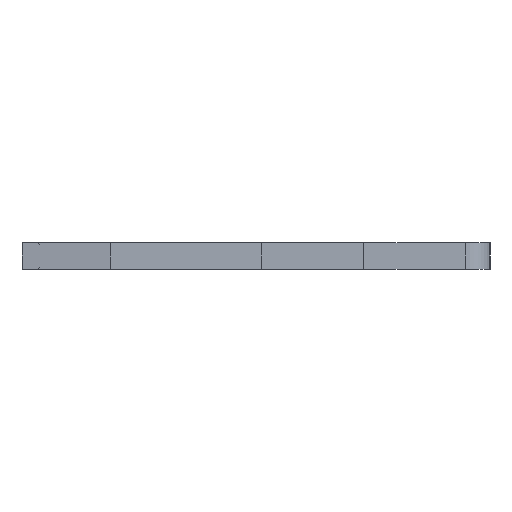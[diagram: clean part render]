
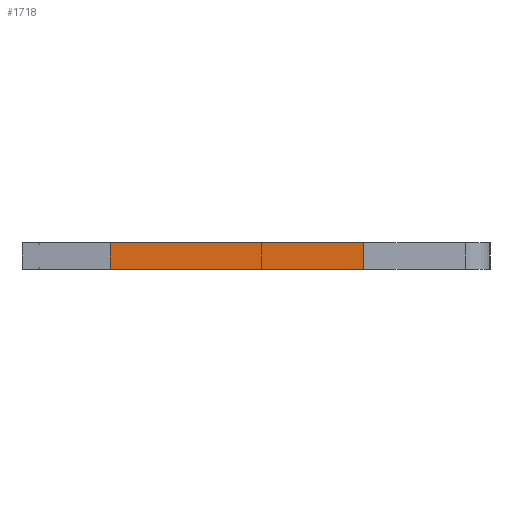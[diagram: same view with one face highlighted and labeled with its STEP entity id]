
A CAD part, left-side view. The second image highlights one B-rep face of the part: STEP entity #1718.
In plain terms, the highlighted face is planar.
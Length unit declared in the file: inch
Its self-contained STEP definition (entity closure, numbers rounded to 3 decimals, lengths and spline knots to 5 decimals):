
#96 = LINE ( 'NONE', #1776, #300 ) ;
#206 = CARTESIAN_POINT ( 'NONE',  ( 0.013, 0.146, -0.0575 ) ) ;
#245 = VECTOR ( 'NONE', #1143, 39.37008 ) ;
#300 = VECTOR ( 'NONE', #1977, 39.37008 ) ;
#362 = CARTESIAN_POINT ( 'NONE',  ( 0.013, -0.099, -0.0575 ) ) ;
#368 = EDGE_CURVE ( 'NONE', #1595, #1169, #1630, .T. ) ;
#499 = PLANE ( 'NONE',  #827 ) ;
#508 = EDGE_LOOP ( 'NONE', ( #2416, #1468, #603, #2275 ) ) ;
#603 = ORIENTED_EDGE ( 'NONE', *, *, #1353, .F. ) ;
#634 = VERTEX_POINT ( 'NONE', #362 ) ;
#827 = AXIS2_PLACEMENT_3D ( 'NONE', #1422, #2082, #1101 ) ;
#872 = LINE ( 'NONE', #206, #2180 ) ;
#1034 = CARTESIAN_POINT ( 'NONE',  ( -0.013, -0.099, -0.0575 ) ) ;
#1045 = CARTESIAN_POINT ( 'NONE',  ( 0.013, 0.146, -0.0575 ) ) ;
#1061 = LINE ( 'NONE', #1045, #1645 ) ;
#1101 = DIRECTION ( 'NONE',  ( 1., 0., 0. ) ) ;
#1143 = DIRECTION ( 'NONE',  ( 0., 1., 0. ) ) ;
#1169 = VERTEX_POINT ( 'NONE', #1210 ) ;
#1210 = CARTESIAN_POINT ( 'NONE',  ( -0.013, 0.146, -0.0575 ) ) ;
#1353 = EDGE_CURVE ( 'NONE', #634, #1444, #872, .T. ) ;
#1422 = CARTESIAN_POINT ( 'NONE',  ( 0.013, 0.146, -0.0575 ) ) ;
#1444 = VERTEX_POINT ( 'NONE', #1594 ) ;
#1468 = ORIENTED_EDGE ( 'NONE', *, *, #1860, .F. ) ;
#1594 = CARTESIAN_POINT ( 'NONE',  ( 0.013, 0.146, -0.0575 ) ) ;
#1595 = VERTEX_POINT ( 'NONE', #1034 ) ;
#1630 = LINE ( 'NONE', #2085, #245 ) ;
#1645 = VECTOR ( 'NONE', #2438, 39.37008 ) ;
#1718 = ADVANCED_FACE ( 'NONE', ( #1735 ), #499, .F. ) ;
#1735 = FACE_OUTER_BOUND ( 'NONE', #508, .T. ) ;
#1776 = CARTESIAN_POINT ( 'NONE',  ( 0.013, -0.099, -0.0575 ) ) ;
#1778 = DIRECTION ( 'NONE',  ( 0., 1., 0. ) ) ;
#1860 = EDGE_CURVE ( 'NONE', #1444, #1169, #1061, .T. ) ;
#1977 = DIRECTION ( 'NONE',  ( -1., 0., 0. ) ) ;
#2082 = DIRECTION ( 'NONE',  ( 0., 0., 1. ) ) ;
#2085 = CARTESIAN_POINT ( 'NONE',  ( -0.013, 0.146, -0.0575 ) ) ;
#2180 = VECTOR ( 'NONE', #1778, 39.37008 ) ;
#2275 = ORIENTED_EDGE ( 'NONE', *, *, #2456, .T. ) ;
#2416 = ORIENTED_EDGE ( 'NONE', *, *, #368, .T. ) ;
#2438 = DIRECTION ( 'NONE',  ( -1., 0., 0. ) ) ;
#2456 = EDGE_CURVE ( 'NONE', #634, #1595, #96, .T. ) ;
